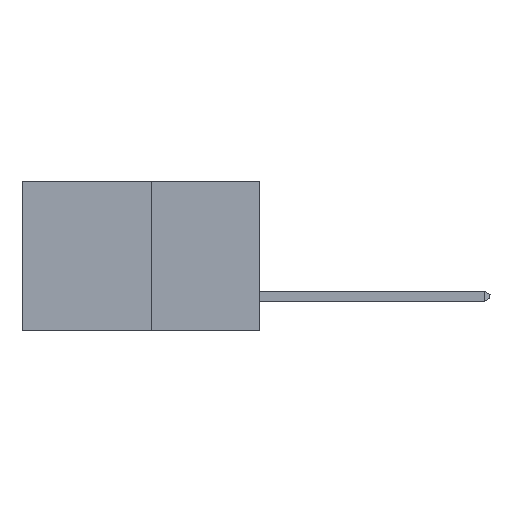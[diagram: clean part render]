
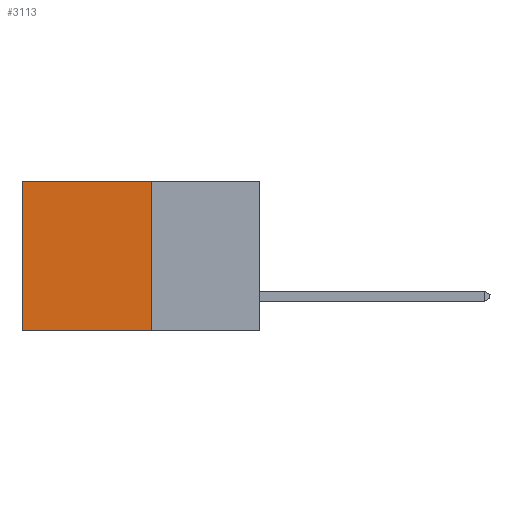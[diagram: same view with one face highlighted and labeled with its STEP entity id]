
A CAD part, left-side view. The second image highlights one B-rep face of the part: STEP entity #3113.
In plain terms, the highlighted planar face has unit normal (-1, 0, 0).
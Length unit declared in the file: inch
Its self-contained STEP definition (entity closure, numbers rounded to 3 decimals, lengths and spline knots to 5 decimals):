
#279 = CARTESIAN_POINT ( 'NONE',  ( 0.277, 0.27, -0.37 ) ) ;
#1975 = CARTESIAN_POINT ( 'NONE',  ( 0.277, 0.59, -0.37 ) ) ;
#2562 = DIRECTION ( 'NONE',  ( 0., 0., -1. ) ) ;
#2843 = EDGE_CURVE ( 'NONE', #23216, #15659, #28801, .T. ) ;
#3113 = ADVANCED_FACE ( 'NONE', ( #19273 ), #17882, .F. ) ;
#3376 = CARTESIAN_POINT ( 'NONE',  ( 0.277, 0.27, 0. ) ) ;
#3496 = CARTESIAN_POINT ( 'NONE',  ( 0.277, 0.59, 0. ) ) ;
#3600 = DIRECTION ( 'NONE',  ( 0., 1., 0. ) ) ;
#5798 = AXIS2_PLACEMENT_3D ( 'NONE', #21205, #21094, #2562 ) ;
#6139 = EDGE_CURVE ( 'NONE', #28918, #11916, #6350, .T. ) ;
#6350 = LINE ( 'NONE', #279, #11585 ) ;
#6933 = VECTOR ( 'NONE', #7552, 39.37008 ) ;
#7552 = DIRECTION ( 'NONE',  ( 0., 0., -1. ) ) ;
#8417 = VECTOR ( 'NONE', #3600, 39.37008 ) ;
#9678 = EDGE_CURVE ( 'NONE', #23216, #28918, #27330, .T. ) ;
#9880 = CARTESIAN_POINT ( 'NONE',  ( 0.277, 0.59, -0.37 ) ) ;
#11390 = CARTESIAN_POINT ( 'NONE',  ( 0.277, 0.27, 0. ) ) ;
#11585 = VECTOR ( 'NONE', #15760, 39.37008 ) ;
#11916 = VERTEX_POINT ( 'NONE', #1975 ) ;
#15659 = VERTEX_POINT ( 'NONE', #3496 ) ;
#15760 = DIRECTION ( 'NONE',  ( 0., 1., 0. ) ) ;
#16200 = VECTOR ( 'NONE', #25188, 39.37008 ) ;
#17882 = PLANE ( 'NONE',  #5798 ) ;
#18162 = EDGE_LOOP ( 'NONE', ( #24634, #23056, #21555, #29595 ) ) ;
#19273 = FACE_OUTER_BOUND ( 'NONE', #18162, .T. ) ;
#21094 = DIRECTION ( 'NONE',  ( 1., 0., 0. ) ) ;
#21205 = CARTESIAN_POINT ( 'NONE',  ( 0.277, 0.27, -0.37 ) ) ;
#21555 = ORIENTED_EDGE ( 'NONE', *, *, #9678, .F. ) ;
#22875 = CARTESIAN_POINT ( 'NONE',  ( 0.277, 0.27, -0.37 ) ) ;
#22930 = LINE ( 'NONE', #9880, #16200 ) ;
#23056 = ORIENTED_EDGE ( 'NONE', *, *, #6139, .F. ) ;
#23216 = VERTEX_POINT ( 'NONE', #11390 ) ;
#23546 = CARTESIAN_POINT ( 'NONE',  ( 0.277, 0.27, -0.37 ) ) ;
#24634 = ORIENTED_EDGE ( 'NONE', *, *, #27342, .T. ) ;
#25188 = DIRECTION ( 'NONE',  ( 0., 0., -1. ) ) ;
#27330 = LINE ( 'NONE', #22875, #6933 ) ;
#27342 = EDGE_CURVE ( 'NONE', #15659, #11916, #22930, .T. ) ;
#28801 = LINE ( 'NONE', #3376, #8417 ) ;
#28918 = VERTEX_POINT ( 'NONE', #23546 ) ;
#29595 = ORIENTED_EDGE ( 'NONE', *, *, #2843, .T. ) ;
